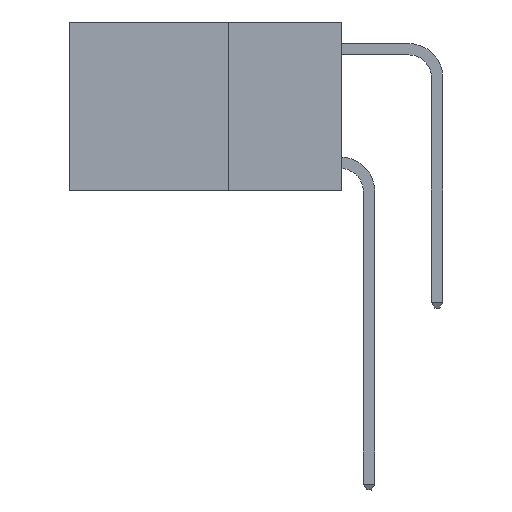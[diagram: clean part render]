
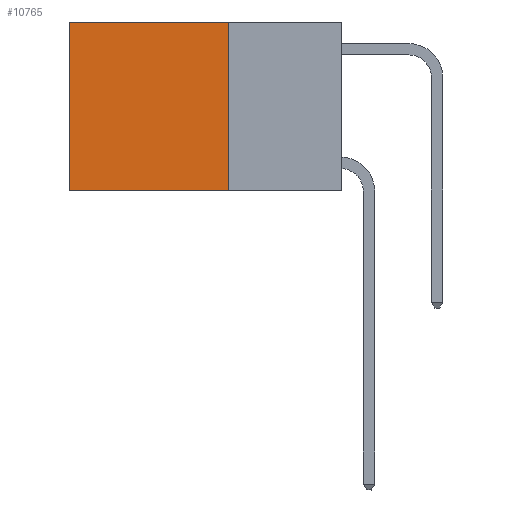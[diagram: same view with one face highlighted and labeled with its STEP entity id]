
A CAD part, left-side view. The second image highlights one B-rep face of the part: STEP entity #10765.
In plain terms, the highlighted planar face has unit normal (-1, 0, 0).
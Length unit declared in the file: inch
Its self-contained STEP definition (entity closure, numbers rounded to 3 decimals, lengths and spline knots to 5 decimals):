
#2017 = CARTESIAN_POINT ( 'NONE',  ( 0.2625, 0.25, 0. ) ) ;
#2024 = DIRECTION ( 'NONE',  ( 0., 0., -1. ) ) ;
#2081 = CARTESIAN_POINT ( 'NONE',  ( 0.2625, 0.6, 0. ) ) ;
#2102 = CARTESIAN_POINT ( 'NONE',  ( 0.2625, 0.25, 0. ) ) ;
#2668 = CARTESIAN_POINT ( 'NONE',  ( 0.2625, 0.25, -0.37 ) ) ;
#3006 = LINE ( 'NONE', #2081, #13301 ) ;
#4761 = VECTOR ( 'NONE', #2024, 39.37008 ) ;
#7266 = ORIENTED_EDGE ( 'NONE', *, *, #9391, .F. ) ;
#8386 = VERTEX_POINT ( 'NONE', #20601 ) ;
#8714 = EDGE_LOOP ( 'NONE', ( #21627, #17368, #7266, #9473 ) ) ;
#8855 = VECTOR ( 'NONE', #15693, 39.37008 ) ;
#9168 = LINE ( 'NONE', #13777, #8855 ) ;
#9391 = EDGE_CURVE ( 'NONE', #14523, #10053, #16812, .T. ) ;
#9473 = ORIENTED_EDGE ( 'NONE', *, *, #12087, .T. ) ;
#10053 = VERTEX_POINT ( 'NONE', #2668 ) ;
#10181 = VERTEX_POINT ( 'NONE', #12198 ) ;
#10765 = ADVANCED_FACE ( 'NONE', ( #15210 ), #12954, .F. ) ;
#11159 = CARTESIAN_POINT ( 'NONE',  ( 0.2625, 0.25, 0. ) ) ;
#11244 = DIRECTION ( 'NONE',  ( 0., 0., -1. ) ) ;
#12087 = EDGE_CURVE ( 'NONE', #14523, #8386, #15708, .T. ) ;
#12198 = CARTESIAN_POINT ( 'NONE',  ( 0.2625, 0.6, -0.37 ) ) ;
#12954 = PLANE ( 'NONE',  #16765 ) ;
#13165 = EDGE_CURVE ( 'NONE', #8386, #10181, #3006, .T. ) ;
#13301 = VECTOR ( 'NONE', #17087, 39.37008 ) ;
#13777 = CARTESIAN_POINT ( 'NONE',  ( 0.2625, 0.25, -0.37 ) ) ;
#14523 = VERTEX_POINT ( 'NONE', #2017 ) ;
#15210 = FACE_OUTER_BOUND ( 'NONE', #8714, .T. ) ;
#15693 = DIRECTION ( 'NONE',  ( 0., 1., 0. ) ) ;
#15708 = LINE ( 'NONE', #17444, #21837 ) ;
#15879 = DIRECTION ( 'NONE',  ( 0., 1., 0. ) ) ;
#16765 = AXIS2_PLACEMENT_3D ( 'NONE', #11159, #19289, #11244 ) ;
#16812 = LINE ( 'NONE', #2102, #4761 ) ;
#17087 = DIRECTION ( 'NONE',  ( 0., 0., -1. ) ) ;
#17368 = ORIENTED_EDGE ( 'NONE', *, *, #22562, .F. ) ;
#17444 = CARTESIAN_POINT ( 'NONE',  ( 0.2625, 0.25, 0. ) ) ;
#19289 = DIRECTION ( 'NONE',  ( 1., 0., 0. ) ) ;
#20601 = CARTESIAN_POINT ( 'NONE',  ( 0.2625, 0.6, 0. ) ) ;
#21627 = ORIENTED_EDGE ( 'NONE', *, *, #13165, .T. ) ;
#21837 = VECTOR ( 'NONE', #15879, 39.37008 ) ;
#22562 = EDGE_CURVE ( 'NONE', #10053, #10181, #9168, .T. ) ;
